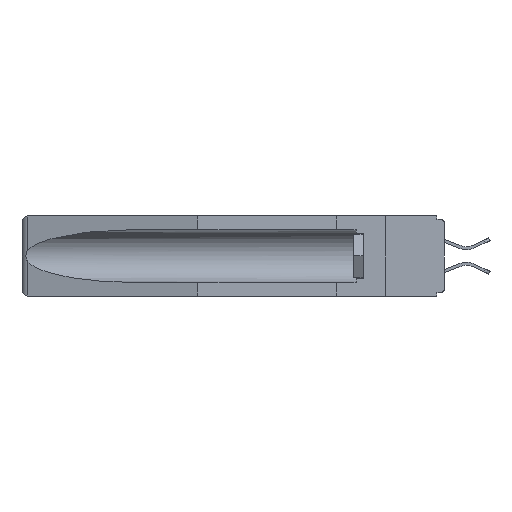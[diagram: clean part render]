
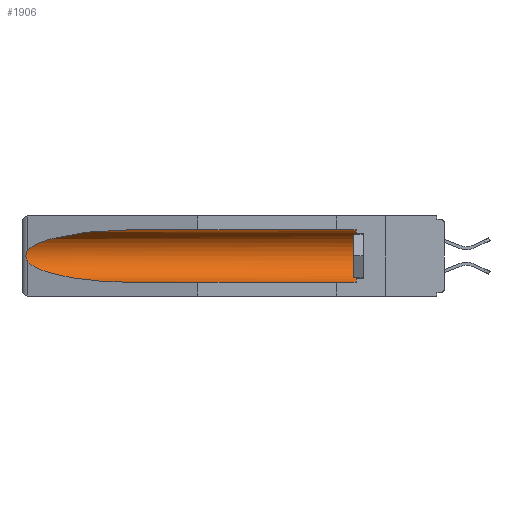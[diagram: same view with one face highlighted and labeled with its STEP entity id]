
A CAD part, left-side view. The second image highlights one B-rep face of the part: STEP entity #1906.
In plain terms, the highlighted cylindrical face has radius 2.857 mm (diameter 5.715 mm), a partial arc.
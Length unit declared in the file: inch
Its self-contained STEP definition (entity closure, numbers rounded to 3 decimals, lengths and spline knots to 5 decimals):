
#431 = CARTESIAN_POINT ( 'NONE',  ( 0.155, -0.30754, -0.284 ) ) ;
#1116 = DIRECTION ( 'NONE',  ( 0., 0., 1. ) ) ;
#1449 = CARTESIAN_POINT ( 'NONE',  ( 0.26537, 1.52718, -0.14972 ) ) ;
#1906 = ADVANCED_FACE ( 'NONE', ( #21992 ), #5981, .F. ) ;
#2090 = ORIENTED_EDGE ( 'NONE', *, *, #3118, .T. ) ;
#2437 = CARTESIAN_POINT ( 'NONE',  ( 0.26537, 1.52718, -0.19328 ) ) ;
#3118 = EDGE_CURVE ( 'NONE', #16615, #11995, #14836, .T. ) ;
#3272 = CARTESIAN_POINT ( 'NONE',  ( 0.155, 1.07973, -0.284 ) ) ;
#4195 = EDGE_CURVE ( 'NONE', #19971, #8868, #16191, .T. ) ;
#4273 = CARTESIAN_POINT ( 'NONE',  ( 0.26597, 1.52961, -0.15275 ) ) ;
#4325 = AXIS2_PLACEMENT_3D ( 'NONE', #17978, #10420, #1116 ) ;
#5981 = CYLINDRICAL_SURFACE ( 'NONE', #4325, 0.1125 ) ;
#6015 = DIRECTION ( 'NONE',  ( 0., -1., 0. ) ) ;
#6075 = VERTEX_POINT ( 'NONE', #7962 ) ;
#6277 = VECTOR ( 'NONE', #13025, 39.37008 ) ;
#6287 = CARTESIAN_POINT ( 'NONE',  ( 0.26537, 1.52718, -0.14972 ) ) ;
#6453 = EDGE_CURVE ( 'NONE', #11995, #23569, #22872, .T. ) ;
#6790 = ORIENTED_EDGE ( 'NONE', *, *, #6453, .T. ) ;
#7197 = CARTESIAN_POINT ( 'NONE',  ( 0.155, 1.07973, -0.284 ) ) ;
#7440 = ORIENTED_EDGE ( 'NONE', *, *, #18296, .T. ) ;
#7962 = CARTESIAN_POINT ( 'NONE',  ( 0.155, 0.126, -0.284 ) ) ;
#8107 =( BOUNDED_CURVE ( )  B_SPLINE_CURVE ( 3, ( #19862, #23829, #8874, #1449 ),
 .UNSPECIFIED., .F., .F. ) 
 B_SPLINE_CURVE_WITH_KNOTS ( ( 4, 4 ),
 ( 4.71239, 6.08839 ),
 .UNSPECIFIED. ) 
 CURVE ( )  GEOMETRIC_REPRESENTATION_ITEM ( )  RATIONAL_B_SPLINE_CURVE ( ( 1., 0.848, 0.848, 1. ) ) 
 REPRESENTATION_ITEM ( '' )  );
#8868 = VERTEX_POINT ( 'NONE', #11828 ) ;
#8874 = CARTESIAN_POINT ( 'NONE',  ( 0.25451, 1.48313, -0.09465 ) ) ;
#9334 = CARTESIAN_POINT ( 'NONE',  ( 0.25451, 1.48313, -0.24835 ) ) ;
#9824 = AXIS2_PLACEMENT_3D ( 'NONE', #22712, #6015, #20523 ) ;
#9841 = DIRECTION ( 'NONE',  ( 0., 1., 0. ) ) ;
#10420 = DIRECTION ( 'NONE',  ( 0., 1., 0. ) ) ;
#10884 = EDGE_LOOP ( 'NONE', ( #20705, #2090, #6790, #18004, #7440, #13655 ) ) ;
#11828 = CARTESIAN_POINT ( 'NONE',  ( 0.155, 1.07973, -0.059 ) ) ;
#11995 = VERTEX_POINT ( 'NONE', #2437 ) ;
#12119 = EDGE_CURVE ( 'NONE', #8868, #16615, #8107, .T. ) ;
#12218 = VECTOR ( 'NONE', #9841, 39.37008 ) ;
#12867 = CARTESIAN_POINT ( 'NONE',  ( 0.155, -0.30754, -0.059 ) ) ;
#13025 = DIRECTION ( 'NONE',  ( 0., 1., 0. ) ) ;
#13539 = CARTESIAN_POINT ( 'NONE',  ( 0.26537, 1.52718, -0.19328 ) ) ;
#13655 = ORIENTED_EDGE ( 'NONE', *, *, #4195, .T. ) ;
#13692 = CARTESIAN_POINT ( 'NONE',  ( 0.2673, 1.5327, -0.16383 ) ) ;
#13700 = EDGE_CURVE ( 'NONE', #6075, #23569, #16888, .T. ) ;
#14836 = B_SPLINE_CURVE_WITH_KNOTS ( 'NONE', 3,
 ( #15402, #4273, #17343, #13692, #17428, #21172, #22806, #19058, #15324, #13539 ),
 .UNSPECIFIED., .F., .F.,
 ( 4, 2, 2, 2, 4 ),
 ( 0., 0.00029, 0.00058, 0.00087, 0.00117 ),
 .UNSPECIFIED. ) ;
#14856 = CARTESIAN_POINT ( 'NONE',  ( 0.26537, 1.52718, -0.19328 ) ) ;
#15324 = CARTESIAN_POINT ( 'NONE',  ( 0.26597, 1.5296, -0.19026 ) ) ;
#15402 = CARTESIAN_POINT ( 'NONE',  ( 0.26537, 1.52718, -0.14972 ) ) ;
#16191 = LINE ( 'NONE', #12867, #6277 ) ;
#16615 = VERTEX_POINT ( 'NONE', #6287 ) ;
#16888 = LINE ( 'NONE', #431, #12218 ) ;
#17343 = CARTESIAN_POINT ( 'NONE',  ( 0.26654, 1.53092, -0.15636 ) ) ;
#17428 = CARTESIAN_POINT ( 'NONE',  ( 0.2675, 1.53308, -0.16763 ) ) ;
#17978 = CARTESIAN_POINT ( 'NONE',  ( 0.155, -0.30754, -0.1715 ) ) ;
#18004 = ORIENTED_EDGE ( 'NONE', *, *, #13700, .F. ) ;
#18296 = EDGE_CURVE ( 'NONE', #6075, #19971, #23238, .T. ) ;
#19058 = CARTESIAN_POINT ( 'NONE',  ( 0.26655, 1.53094, -0.18657 ) ) ;
#19862 = CARTESIAN_POINT ( 'NONE',  ( 0.155, 1.07973, -0.059 ) ) ;
#19971 = VERTEX_POINT ( 'NONE', #22868 ) ;
#20523 = DIRECTION ( 'NONE',  ( 0., 0., 1. ) ) ;
#20705 = ORIENTED_EDGE ( 'NONE', *, *, #12119, .T. ) ;
#21172 = CARTESIAN_POINT ( 'NONE',  ( 0.2675, 1.53308, -0.17534 ) ) ;
#21992 = FACE_OUTER_BOUND ( 'NONE', #10884, .T. ) ;
#22329 = CARTESIAN_POINT ( 'NONE',  ( 0.21114, 1.30732, -0.284 ) ) ;
#22712 = CARTESIAN_POINT ( 'NONE',  ( 0.155, 0.126, -0.1715 ) ) ;
#22806 = CARTESIAN_POINT ( 'NONE',  ( 0.2673, 1.53269, -0.17917 ) ) ;
#22868 = CARTESIAN_POINT ( 'NONE',  ( 0.155, 0.126, -0.059 ) ) ;
#22872 =( BOUNDED_CURVE ( )  B_SPLINE_CURVE ( 3, ( #14856, #9334, #22329, #7197 ),
 .UNSPECIFIED., .F., .F. ) 
 B_SPLINE_CURVE_WITH_KNOTS ( ( 4, 4 ),
 ( 0.1948, 1.5708 ),
 .UNSPECIFIED. ) 
 CURVE ( )  GEOMETRIC_REPRESENTATION_ITEM ( )  RATIONAL_B_SPLINE_CURVE ( ( 1., 0.848, 0.848, 1. ) ) 
 REPRESENTATION_ITEM ( '' )  );
#23238 = CIRCLE ( 'NONE', #9824, 0.1125 ) ;
#23569 = VERTEX_POINT ( 'NONE', #3272 ) ;
#23829 = CARTESIAN_POINT ( 'NONE',  ( 0.21114, 1.30732, -0.059 ) ) ;
